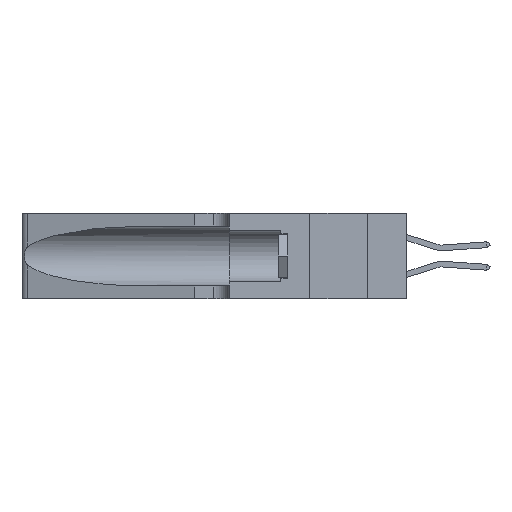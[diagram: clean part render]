
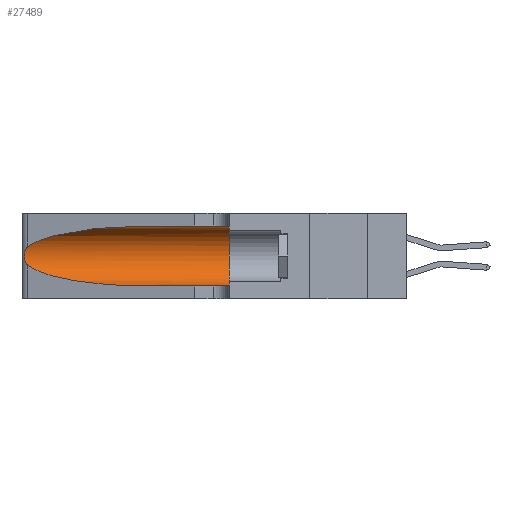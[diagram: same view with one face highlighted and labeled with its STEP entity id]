
A CAD part, left-side view. The second image highlights one B-rep face of the part: STEP entity #27489.
In plain terms, the highlighted cylindrical face has radius 3.308 mm (diameter 6.617 mm), a partial arc.
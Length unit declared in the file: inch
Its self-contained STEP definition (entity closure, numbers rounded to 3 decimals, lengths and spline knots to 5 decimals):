
#82 = EDGE_CURVE ( 'NONE', #12040, #22267, #8111, .T. ) ;
#759 = CARTESIAN_POINT ( 'NONE',  ( 0.25555, 1.22993, 0.14849 ) ) ;
#1079 = VERTEX_POINT ( 'NONE', #27801 ) ;
#1723 = VERTEX_POINT ( 'NONE', #8079 ) ;
#1832 = VECTOR ( 'NONE', #13462, 39.37008 ) ;
#2983 = CIRCLE ( 'NONE', #17644, 0.13025 ) ;
#3919 = CARTESIAN_POINT ( 'NONE',  ( 0.1305, 0.72297, 0.31525 ) ) ;
#5436 = CARTESIAN_POINT ( 'NONE',  ( 0.25787, 1.23484, 0.2124 ) ) ;
#6486 = FACE_OUTER_BOUND ( 'NONE', #29039, .T. ) ;
#6824 = ORIENTED_EDGE ( 'NONE', *, *, #10942, .F. ) ;
#7797 = CARTESIAN_POINT ( 'NONE',  ( 0.26018, 1.23835, 0.19895 ) ) ;
#8079 = CARTESIAN_POINT ( 'NONE',  ( 0.25487, 1.22718, 0.22369 ) ) ;
#8111 = LINE ( 'NONE', #11665, #1832 ) ;
#8735 = EDGE_CURVE ( 'NONE', #1079, #12040, #12088, .T. ) ;
#10264 = CARTESIAN_POINT ( 'NONE',  ( 0.26075, 1.23896, 0.178 ) ) ;
#10689 = EDGE_CURVE ( 'NONE', #22755, #22267, #2983, .T. ) ;
#10942 = EDGE_CURVE ( 'NONE', #21019, #22755, #13704, .T. ) ;
#11126 = CARTESIAN_POINT ( 'NONE',  ( 0.2373, 1.15595, 0.28018 ) ) ;
#11665 = CARTESIAN_POINT ( 'NONE',  ( 0.1305, 1.61858, 0.05475 ) ) ;
#12040 = VERTEX_POINT ( 'NONE', #28303 ) ;
#12048 = CARTESIAN_POINT ( 'NONE',  ( 0.1305, 0.35, 0.185 ) ) ;
#12088 =( BOUNDED_CURVE ( )  B_SPLINE_CURVE ( 3, ( #12905, #26644, #28935, #15202 ),
 .UNSPECIFIED., .F., .F. ) 
 B_SPLINE_CURVE_WITH_KNOTS ( ( 4, 4 ),
 ( 3.44316, 4.71239 ),
 .UNSPECIFIED. ) 
 CURVE ( )  GEOMETRIC_REPRESENTATION_ITEM ( )  RATIONAL_B_SPLINE_CURVE ( ( 1., 0.87, 0.87, 1. ) ) 
 REPRESENTATION_ITEM ( '' )  );
#12177 = CARTESIAN_POINT ( 'NONE',  ( 0.1305, 0.35, 0.05475 ) ) ;
#12619 = CARTESIAN_POINT ( 'NONE',  ( 0.25856, 1.23593, 0.16098 ) ) ;
#12905 = CARTESIAN_POINT ( 'NONE',  ( 0.25487, 1.22718, 0.14631 ) ) ;
#12999 = B_SPLINE_CURVE_WITH_KNOTS ( 'NONE', 3,
 ( #26260, #28556, #19435, #5436, #21745, #7797, #24066, #10264, #26362, #12619, #28661, #14920, #759, #17211 ),
 .UNSPECIFIED., .F., .F.,
 ( 4, 2, 2, 2, 2, 2, 4 ),
 ( 0., 0.00027, 0.00053, 0.00107, 0.0016, 0.00187, 0.00214 ),
 .UNSPECIFIED. ) ;
#13344 = CARTESIAN_POINT ( 'NONE',  ( 0.1305, 1.61858, 0.31525 ) ) ;
#13462 = DIRECTION ( 'NONE',  ( 0., -1., 0. ) ) ;
#13704 = LINE ( 'NONE', #13344, #19810 ) ;
#13854 = DIRECTION ( 'NONE',  ( 0., 0., -1. ) ) ;
#14748 = DIRECTION ( 'NONE',  ( 0., 0., 1. ) ) ;
#14920 = CARTESIAN_POINT ( 'NONE',  ( 0.25639, 1.23186, 0.15144 ) ) ;
#15202 = CARTESIAN_POINT ( 'NONE',  ( 0.1305, 0.72297, 0.05475 ) ) ;
#15730 = ORIENTED_EDGE ( 'NONE', *, *, #10689, .F. ) ;
#17211 = CARTESIAN_POINT ( 'NONE',  ( 0.25487, 1.22718, 0.14631 ) ) ;
#17644 = AXIS2_PLACEMENT_3D ( 'NONE', #12048, #28477, #14748 ) ;
#17999 = EDGE_CURVE ( 'NONE', #21019, #1723, #23651, .T. ) ;
#18200 = CYLINDRICAL_SURFACE ( 'NONE', #20490, 0.13025 ) ;
#18343 = DIRECTION ( 'NONE',  ( 0., -1., 0. ) ) ;
#18360 = EDGE_CURVE ( 'NONE', #1723, #1079, #12999, .T. ) ;
#19435 = CARTESIAN_POINT ( 'NONE',  ( 0.25639, 1.23184, 0.21858 ) ) ;
#19442 = CARTESIAN_POINT ( 'NONE',  ( 0.1305, 0.72297, 0.31525 ) ) ;
#19810 = VECTOR ( 'NONE', #29390, 39.37008 ) ;
#20260 = CARTESIAN_POINT ( 'NONE',  ( 0.18966, 0.96281, 0.31525 ) ) ;
#20490 = AXIS2_PLACEMENT_3D ( 'NONE', #29894, #18343, #13854 ) ;
#21019 = VERTEX_POINT ( 'NONE', #19442 ) ;
#21745 = CARTESIAN_POINT ( 'NONE',  ( 0.25854, 1.2359, 0.20912 ) ) ;
#22136 = ORIENTED_EDGE ( 'NONE', *, *, #17999, .T. ) ;
#22267 = VERTEX_POINT ( 'NONE', #12177 ) ;
#22755 = VERTEX_POINT ( 'NONE', #28618 ) ;
#22981 = ORIENTED_EDGE ( 'NONE', *, *, #8735, .T. ) ;
#23157 = ORIENTED_EDGE ( 'NONE', *, *, #18360, .T. ) ;
#23651 =( BOUNDED_CURVE ( )  B_SPLINE_CURVE ( 3, ( #3919, #20260, #11126, #27188 ),
 .UNSPECIFIED., .F., .T. ) 
 B_SPLINE_CURVE_WITH_KNOTS ( ( 4, 4 ),
 ( 1.5708, 2.84003 ),
 .UNSPECIFIED. ) 
 CURVE ( )  GEOMETRIC_REPRESENTATION_ITEM ( )  RATIONAL_B_SPLINE_CURVE ( ( 1., 0.87, 0.87, 1. ) ) 
 REPRESENTATION_ITEM ( '' )  );
#24066 = CARTESIAN_POINT ( 'NONE',  ( 0.26075, 1.23896, 0.19203 ) ) ;
#26260 = CARTESIAN_POINT ( 'NONE',  ( 0.25487, 1.22718, 0.22369 ) ) ;
#26362 = CARTESIAN_POINT ( 'NONE',  ( 0.26017, 1.23833, 0.17102 ) ) ;
#26644 = CARTESIAN_POINT ( 'NONE',  ( 0.2373, 1.15595, 0.08982 ) ) ;
#27188 = CARTESIAN_POINT ( 'NONE',  ( 0.25487, 1.22718, 0.22369 ) ) ;
#27489 = ADVANCED_FACE ( 'NONE', ( #6486 ), #18200, .F. ) ;
#27801 = CARTESIAN_POINT ( 'NONE',  ( 0.25487, 1.22718, 0.14631 ) ) ;
#28303 = CARTESIAN_POINT ( 'NONE',  ( 0.1305, 0.72297, 0.05475 ) ) ;
#28477 = DIRECTION ( 'NONE',  ( 0., 1., 0. ) ) ;
#28556 = CARTESIAN_POINT ( 'NONE',  ( 0.25555, 1.22994, 0.2215 ) ) ;
#28618 = CARTESIAN_POINT ( 'NONE',  ( 0.1305, 0.35, 0.31525 ) ) ;
#28661 = CARTESIAN_POINT ( 'NONE',  ( 0.25789, 1.23486, 0.15765 ) ) ;
#28684 = ORIENTED_EDGE ( 'NONE', *, *, #82, .T. ) ;
#28935 = CARTESIAN_POINT ( 'NONE',  ( 0.18966, 0.96281, 0.05475 ) ) ;
#29039 = EDGE_LOOP ( 'NONE', ( #22136, #23157, #22981, #28684, #15730, #6824 ) ) ;
#29390 = DIRECTION ( 'NONE',  ( 0., -1., 0. ) ) ;
#29894 = CARTESIAN_POINT ( 'NONE',  ( 0.1305, 1.61858, 0.185 ) ) ;
